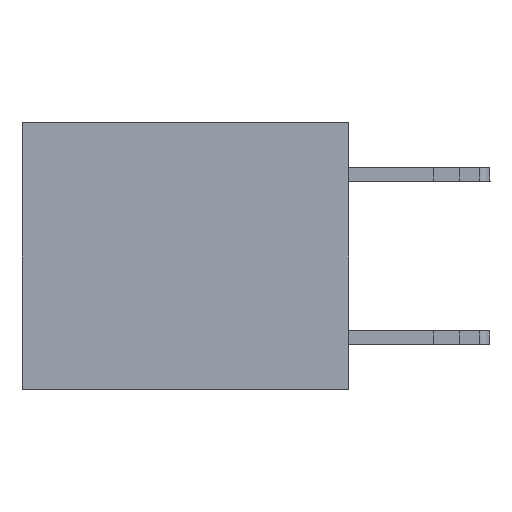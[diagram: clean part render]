
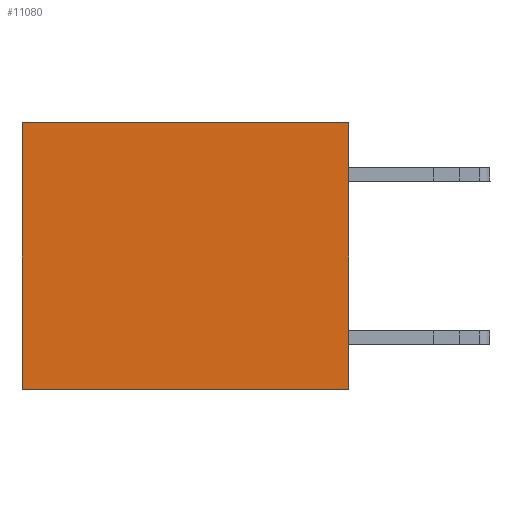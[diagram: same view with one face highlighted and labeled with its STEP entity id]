
A CAD part, left-side view. The second image highlights one B-rep face of the part: STEP entity #11080.
In plain terms, the highlighted planar face has unit normal (-1, 0, 0).
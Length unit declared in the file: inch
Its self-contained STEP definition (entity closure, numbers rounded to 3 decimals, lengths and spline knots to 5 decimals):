
#1066 = CARTESIAN_POINT ( 'NONE',  ( 0.3165, 0.6, 0. ) ) ;
#1948 = EDGE_CURVE ( 'NONE', #7164, #18110, #5226, .T. ) ;
#3544 = VECTOR ( 'NONE', #4230, 39.37008 ) ;
#4230 = DIRECTION ( 'NONE',  ( 0., 0., -1. ) ) ;
#4488 = ORIENTED_EDGE ( 'NONE', *, *, #8190, .T. ) ;
#5226 = LINE ( 'NONE', #11830, #20911 ) ;
#5586 = EDGE_LOOP ( 'NONE', ( #7773, #11880, #12031, #4488 ) ) ;
#5849 = LINE ( 'NONE', #17564, #13683 ) ;
#5899 = CARTESIAN_POINT ( 'NONE',  ( 0.3165, 0., -0.49 ) ) ;
#6066 = EDGE_CURVE ( 'NONE', #18110, #10792, #14572, .T. ) ;
#7164 = VERTEX_POINT ( 'NONE', #10809 ) ;
#7773 = ORIENTED_EDGE ( 'NONE', *, *, #20754, .T. ) ;
#8190 = EDGE_CURVE ( 'NONE', #7164, #15879, #5849, .T. ) ;
#8300 = VECTOR ( 'NONE', #12295, 39.37008 ) ;
#9361 = CARTESIAN_POINT ( 'NONE',  ( 0.3165, 0.6, -0.49 ) ) ;
#10792 = VERTEX_POINT ( 'NONE', #17802 ) ;
#10809 = CARTESIAN_POINT ( 'NONE',  ( 0.3165, 0., 0. ) ) ;
#11080 = ADVANCED_FACE ( 'NONE', ( #16454 ), #16020, .F. ) ;
#11830 = CARTESIAN_POINT ( 'NONE',  ( 0.3165, 0., -0.49 ) ) ;
#11880 = ORIENTED_EDGE ( 'NONE', *, *, #6066, .F. ) ;
#12031 = ORIENTED_EDGE ( 'NONE', *, *, #1948, .F. ) ;
#12295 = DIRECTION ( 'NONE',  ( 0., 1., 0. ) ) ;
#12429 = CARTESIAN_POINT ( 'NONE',  ( 0.3165, 0., -0.49 ) ) ;
#13516 = DIRECTION ( 'NONE',  ( 0., 0., -1. ) ) ;
#13683 = VECTOR ( 'NONE', #20801, 39.37008 ) ;
#14094 = AXIS2_PLACEMENT_3D ( 'NONE', #5899, #15871, #17567 ) ;
#14572 = LINE ( 'NONE', #12429, #8300 ) ;
#15871 = DIRECTION ( 'NONE',  ( 1., 0., 0. ) ) ;
#15879 = VERTEX_POINT ( 'NONE', #1066 ) ;
#16020 = PLANE ( 'NONE',  #14094 ) ;
#16454 = FACE_OUTER_BOUND ( 'NONE', #5586, .T. ) ;
#17564 = CARTESIAN_POINT ( 'NONE',  ( 0.3165, 0., 0. ) ) ;
#17567 = DIRECTION ( 'NONE',  ( 0., 0., -1. ) ) ;
#17802 = CARTESIAN_POINT ( 'NONE',  ( 0.3165, 0.6, -0.49 ) ) ;
#18110 = VERTEX_POINT ( 'NONE', #18272 ) ;
#18272 = CARTESIAN_POINT ( 'NONE',  ( 0.3165, 0., -0.49 ) ) ;
#18973 = LINE ( 'NONE', #9361, #3544 ) ;
#20754 = EDGE_CURVE ( 'NONE', #15879, #10792, #18973, .T. ) ;
#20801 = DIRECTION ( 'NONE',  ( 0., 1., 0. ) ) ;
#20911 = VECTOR ( 'NONE', #13516, 39.37008 ) ;
